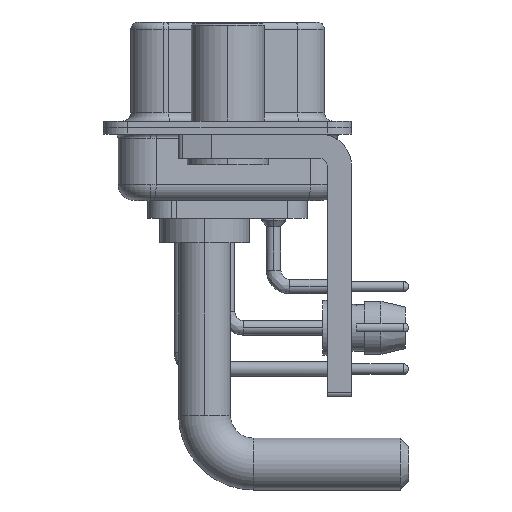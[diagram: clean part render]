
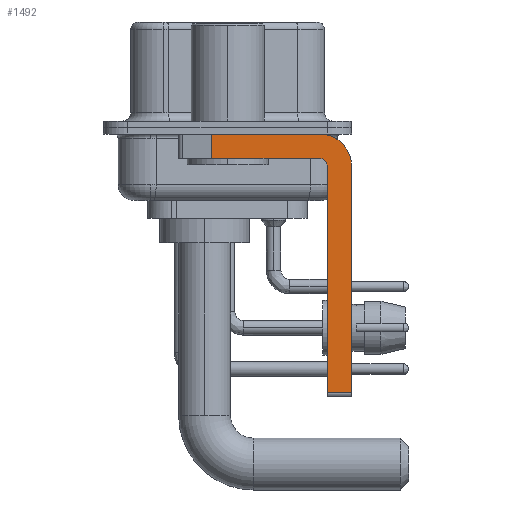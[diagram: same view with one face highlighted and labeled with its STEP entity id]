
A CAD part, left-side view. The second image highlights one B-rep face of the part: STEP entity #1492.
In plain terms, the highlighted planar face has unit normal (-1, 0, 0).
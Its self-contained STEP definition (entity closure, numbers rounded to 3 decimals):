
#257 = FACE_OUTER_BOUND ( 'NONE', #3597, .T. ) ;
#570 = DIRECTION ( 'NONE',  ( 0., 0., -1. ) ) ;
#1142 = VECTOR ( 'NONE', #570, 1000. ) ;
#1492 = ADVANCED_FACE ( 'NONE', ( #257 ), #21412, .F. ) ;
#1558 = DIRECTION ( 'NONE',  ( 0., 0., 1. ) ) ;
#1587 = VERTEX_POINT ( 'NONE', #16731 ) ;
#1749 = CARTESIAN_POINT ( 'NONE',  ( -2.9, -5.65, -1.9 ) ) ;
#2244 = EDGE_CURVE ( 'NONE', #9707, #35286, #13940, .T. ) ;
#3081 = EDGE_CURVE ( 'NONE', #21370, #9707, #23914, .T. ) ;
#3597 = EDGE_LOOP ( 'NONE', ( #36659, #21942, #38203, #4595, #5856, #9666, #22095, #7465 ) ) ;
#4189 = CARTESIAN_POINT ( 'NONE',  ( -2.9, -5.65, -2.4 ) ) ;
#4210 = AXIS2_PLACEMENT_3D ( 'NONE', #4189, #33858, #24956 ) ;
#4595 = ORIENTED_EDGE ( 'NONE', *, *, #20153, .F. ) ;
#4957 = CARTESIAN_POINT ( 'NONE',  ( -2.9, -5.65, -16.35 ) ) ;
#5575 = EDGE_CURVE ( 'NONE', #22825, #17241, #11404, .T. ) ;
#5856 = ORIENTED_EDGE ( 'NONE', *, *, #33156, .F. ) ;
#7465 = ORIENTED_EDGE ( 'NONE', *, *, #2244, .F. ) ;
#7932 = CIRCLE ( 'NONE', #4210, 0.5 ) ;
#9256 = CARTESIAN_POINT ( 'NONE',  ( -2.9, -7.65, -2.4 ) ) ;
#9666 = ORIENTED_EDGE ( 'NONE', *, *, #32762, .T. ) ;
#9707 = VERTEX_POINT ( 'NONE', #31963 ) ;
#10132 = VECTOR ( 'NONE', #34061, 1000. ) ;
#11404 = LINE ( 'NONE', #13715, #10132 ) ;
#12241 = CARTESIAN_POINT ( 'NONE',  ( -2.9, -7.65, -16.35 ) ) ;
#13715 = CARTESIAN_POINT ( 'NONE',  ( -2.9, -5.65, -1.9 ) ) ;
#13940 = CIRCLE ( 'NONE', #28804, 2. ) ;
#14341 = DIRECTION ( 'NONE',  ( 0., 0., -1. ) ) ;
#14897 = CARTESIAN_POINT ( 'NONE',  ( -2.9, 0.978, -0.4 ) ) ;
#15584 = DIRECTION ( 'NONE',  ( 0., 0., -1. ) ) ;
#16334 = LINE ( 'NONE', #33769, #36619 ) ;
#16731 = CARTESIAN_POINT ( 'NONE',  ( -2.9, -6.15, -2.4 ) ) ;
#17241 = VERTEX_POINT ( 'NONE', #28185 ) ;
#19406 = AXIS2_PLACEMENT_3D ( 'NONE', #21601, #33236, #15584 ) ;
#20153 = EDGE_CURVE ( 'NONE', #1587, #22825, #7932, .T. ) ;
#20572 = VERTEX_POINT ( 'NONE', #12241 ) ;
#20929 = LINE ( 'NONE', #32939, #32906 ) ;
#21370 = VERTEX_POINT ( 'NONE', #14897 ) ;
#21412 = PLANE ( 'NONE',  #19406 ) ;
#21601 = CARTESIAN_POINT ( 'NONE',  ( -2.9, -5.65, -2.4 ) ) ;
#21942 = ORIENTED_EDGE ( 'NONE', *, *, #30445, .T. ) ;
#22095 = ORIENTED_EDGE ( 'NONE', *, *, #24681, .F. ) ;
#22825 = VERTEX_POINT ( 'NONE', #1749 ) ;
#23914 = LINE ( 'NONE', #33007, #30679 ) ;
#24681 = EDGE_CURVE ( 'NONE', #35286, #20572, #20929, .T. ) ;
#24956 = DIRECTION ( 'NONE',  ( 0., 0., 1. ) ) ;
#25515 = LINE ( 'NONE', #4957, #33521 ) ;
#27159 = LINE ( 'NONE', #34235, #1142 ) ;
#27274 = DIRECTION ( 'NONE',  ( 0., 0., -1. ) ) ;
#28153 = CARTESIAN_POINT ( 'NONE',  ( -2.9, -6.15, -16.35 ) ) ;
#28185 = CARTESIAN_POINT ( 'NONE',  ( -2.9, 0.978, -1.9 ) ) ;
#28273 = VERTEX_POINT ( 'NONE', #28153 ) ;
#28804 = AXIS2_PLACEMENT_3D ( 'NONE', #33464, #36379, #27274 ) ;
#30445 = EDGE_CURVE ( 'NONE', #21370, #17241, #27159, .T. ) ;
#30679 = VECTOR ( 'NONE', #35715, 1000. ) ;
#31963 = CARTESIAN_POINT ( 'NONE',  ( -2.9, -5.65, -0.4 ) ) ;
#32762 = EDGE_CURVE ( 'NONE', #28273, #20572, #25515, .T. ) ;
#32906 = VECTOR ( 'NONE', #14341, 1000. ) ;
#32939 = CARTESIAN_POINT ( 'NONE',  ( -2.9, -7.65, -2.4 ) ) ;
#33007 = CARTESIAN_POINT ( 'NONE',  ( -2.9, 3., -0.4 ) ) ;
#33156 = EDGE_CURVE ( 'NONE', #28273, #1587, #16334, .T. ) ;
#33236 = DIRECTION ( 'NONE',  ( 1., 0., 0. ) ) ;
#33464 = CARTESIAN_POINT ( 'NONE',  ( -2.9, -5.65, -2.4 ) ) ;
#33521 = VECTOR ( 'NONE', #34238, 1000. ) ;
#33769 = CARTESIAN_POINT ( 'NONE',  ( -2.9, -6.15, -16.6 ) ) ;
#33858 = DIRECTION ( 'NONE',  ( -1., 0., 0. ) ) ;
#34061 = DIRECTION ( 'NONE',  ( 0., 1., 0. ) ) ;
#34235 = CARTESIAN_POINT ( 'NONE',  ( -2.9, 0.978, -1.9 ) ) ;
#34238 = DIRECTION ( 'NONE',  ( 0., -1., 0. ) ) ;
#35286 = VERTEX_POINT ( 'NONE', #9256 ) ;
#35715 = DIRECTION ( 'NONE',  ( 0., -1., 0. ) ) ;
#36379 = DIRECTION ( 'NONE',  ( 1., 0., 0. ) ) ;
#36619 = VECTOR ( 'NONE', #1558, 1000. ) ;
#36659 = ORIENTED_EDGE ( 'NONE', *, *, #3081, .F. ) ;
#38203 = ORIENTED_EDGE ( 'NONE', *, *, #5575, .F. ) ;
